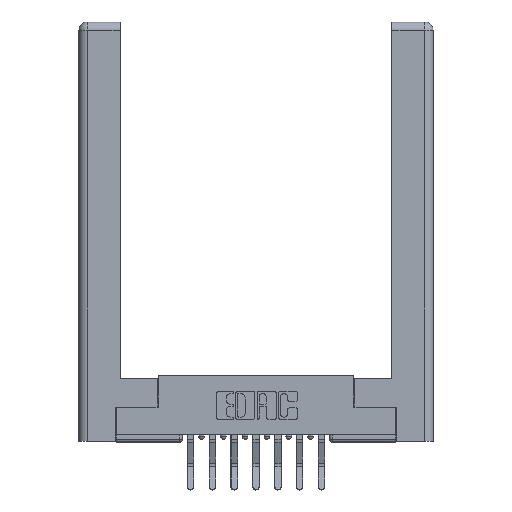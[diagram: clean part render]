
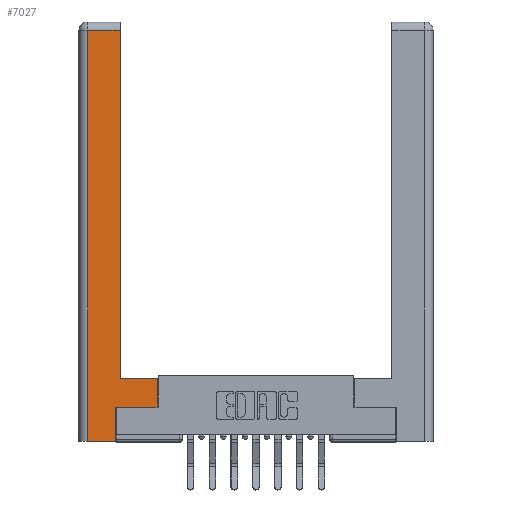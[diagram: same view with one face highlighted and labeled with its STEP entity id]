
A CAD part, top view. The second image highlights one B-rep face of the part: STEP entity #7027.
In plain terms, the highlighted planar face has unit normal (0, 0, 1).
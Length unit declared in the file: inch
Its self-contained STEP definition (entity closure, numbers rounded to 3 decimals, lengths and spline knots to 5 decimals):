
#355 = LINE ( 'NONE', #6526, #8131 ) ;
#455 = VERTEX_POINT ( 'NONE', #4739 ) ;
#493 = VECTOR ( 'NONE', #8066, 39.37008 ) ;
#1252 = DIRECTION ( 'NONE',  ( 0., 1., 0. ) ) ;
#1289 = DIRECTION ( 'NONE',  ( 0., 1., 0. ) ) ;
#1339 = CARTESIAN_POINT ( 'NONE',  ( 0.295, 0.45, 0. ) ) ;
#1459 = CARTESIAN_POINT ( 'NONE',  ( 0.265, 0.245, 0. ) ) ;
#1497 = DIRECTION ( 'NONE',  ( 1., 0., 0. ) ) ;
#1501 = DIRECTION ( 'NONE',  ( -1., 0., 0. ) ) ;
#1510 = EDGE_LOOP ( 'NONE', ( #11709, #11476, #11874, #6315, #4481, #7593, #4659, #8402 ) ) ;
#1889 = DIRECTION ( 'NONE',  ( 0., -1., 0. ) ) ;
#1927 = EDGE_CURVE ( 'NONE', #10214, #1979, #3020, .T. ) ;
#1979 = VERTEX_POINT ( 'NONE', #12476 ) ;
#2387 = CARTESIAN_POINT ( 'NONE',  ( 0.0615, 2.94, 0. ) ) ;
#2814 = EDGE_CURVE ( 'NONE', #1979, #455, #355, .T. ) ;
#3020 = LINE ( 'NONE', #13034, #9832 ) ;
#3078 = CARTESIAN_POINT ( 'NONE',  ( 0.295, 2.94, 0. ) ) ;
#3222 = AXIS2_PLACEMENT_3D ( 'NONE', #3531, #5776, #1501 ) ;
#3516 = VECTOR ( 'NONE', #1252, 39.37008 ) ;
#3531 = CARTESIAN_POINT ( 'NONE',  ( 0., 0., 0. ) ) ;
#3568 = LINE ( 'NONE', #9894, #4591 ) ;
#3782 = CARTESIAN_POINT ( 'NONE',  ( 0.565, 0.45, 0. ) ) ;
#4240 = CARTESIAN_POINT ( 'NONE',  ( 0.295, 3., 0. ) ) ;
#4481 = ORIENTED_EDGE ( 'NONE', *, *, #13028, .T. ) ;
#4591 = VECTOR ( 'NONE', #9753, 39.37008 ) ;
#4659 = ORIENTED_EDGE ( 'NONE', *, *, #5380, .T. ) ;
#4739 = CARTESIAN_POINT ( 'NONE',  ( 0.265, 0., 0. ) ) ;
#5380 = EDGE_CURVE ( 'NONE', #10944, #7090, #7487, .T. ) ;
#5477 = DIRECTION ( 'NONE',  ( 0., 1., 0. ) ) ;
#5634 = DIRECTION ( 'NONE',  ( -1., 0., 0. ) ) ;
#5686 = VECTOR ( 'NONE', #1289, 39.37008 ) ;
#5776 = DIRECTION ( 'NONE',  ( 0., 0., -1. ) ) ;
#6193 = EDGE_CURVE ( 'NONE', #12679, #9538, #12321, .T. ) ;
#6315 = ORIENTED_EDGE ( 'NONE', *, *, #2814, .T. ) ;
#6320 = VECTOR ( 'NONE', #5477, 39.37008 ) ;
#6360 = LINE ( 'NONE', #1459, #6320 ) ;
#6526 = CARTESIAN_POINT ( 'NONE',  ( 0.265, 0., 0. ) ) ;
#6792 = VERTEX_POINT ( 'NONE', #12128 ) ;
#7027 = ADVANCED_FACE ( 'NONE', ( #12991 ), #9850, .F. ) ;
#7050 = LINE ( 'NONE', #12312, #493 ) ;
#7090 = VERTEX_POINT ( 'NONE', #3782 ) ;
#7487 = LINE ( 'NONE', #10408, #3516 ) ;
#7593 = ORIENTED_EDGE ( 'NONE', *, *, #12772, .T. ) ;
#7729 = VECTOR ( 'NONE', #5634, 39.37008 ) ;
#8066 = DIRECTION ( 'NONE',  ( -1., 0., 0. ) ) ;
#8131 = VECTOR ( 'NONE', #1497, 39.37008 ) ;
#8402 = ORIENTED_EDGE ( 'NONE', *, *, #10564, .T. ) ;
#8688 = LINE ( 'NONE', #9574, #7729 ) ;
#9538 = VERTEX_POINT ( 'NONE', #3078 ) ;
#9574 = CARTESIAN_POINT ( 'NONE',  ( 0.295, 0.45, 0. ) ) ;
#9753 = DIRECTION ( 'NONE',  ( 1., 0., 0. ) ) ;
#9832 = VECTOR ( 'NONE', #1889, 39.37008 ) ;
#9850 = PLANE ( 'NONE',  #3222 ) ;
#9894 = CARTESIAN_POINT ( 'NONE',  ( 0.565, 0.245, 0. ) ) ;
#10214 = VERTEX_POINT ( 'NONE', #2387 ) ;
#10408 = CARTESIAN_POINT ( 'NONE',  ( 0.565, 0.45, 0. ) ) ;
#10564 = EDGE_CURVE ( 'NONE', #7090, #12679, #8688, .T. ) ;
#10944 = VERTEX_POINT ( 'NONE', #11353 ) ;
#11353 = CARTESIAN_POINT ( 'NONE',  ( 0.565, 0.245, 0. ) ) ;
#11476 = ORIENTED_EDGE ( 'NONE', *, *, #12514, .T. ) ;
#11709 = ORIENTED_EDGE ( 'NONE', *, *, #6193, .T. ) ;
#11874 = ORIENTED_EDGE ( 'NONE', *, *, #1927, .T. ) ;
#12128 = CARTESIAN_POINT ( 'NONE',  ( 0.265, 0.245, 0. ) ) ;
#12312 = CARTESIAN_POINT ( 'NONE',  ( 0.0615, 2.94, 0. ) ) ;
#12321 = LINE ( 'NONE', #4240, #5686 ) ;
#12476 = CARTESIAN_POINT ( 'NONE',  ( 0.0615, 0., 0. ) ) ;
#12514 = EDGE_CURVE ( 'NONE', #9538, #10214, #7050, .T. ) ;
#12679 = VERTEX_POINT ( 'NONE', #1339 ) ;
#12772 = EDGE_CURVE ( 'NONE', #6792, #10944, #3568, .T. ) ;
#12991 = FACE_OUTER_BOUND ( 'NONE', #1510, .T. ) ;
#13028 = EDGE_CURVE ( 'NONE', #455, #6792, #6360, .T. ) ;
#13034 = CARTESIAN_POINT ( 'NONE',  ( 0.0615, 0., 0. ) ) ;
